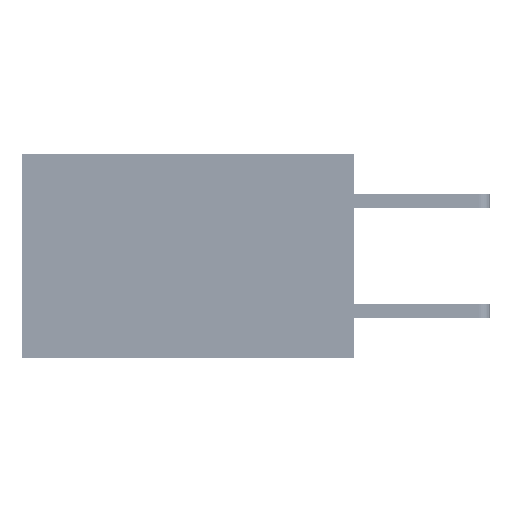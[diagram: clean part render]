
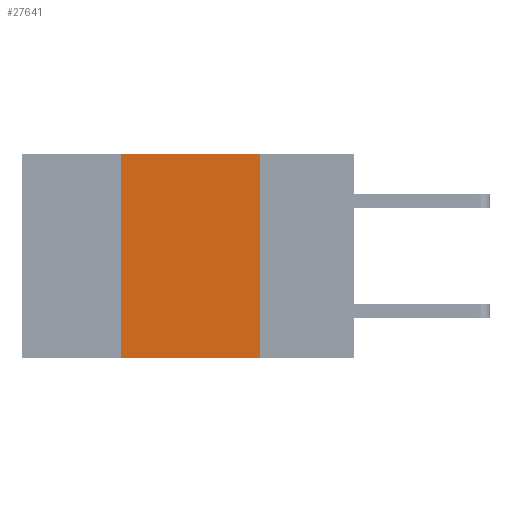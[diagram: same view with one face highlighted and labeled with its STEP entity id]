
A CAD part, left-side view. The second image highlights one B-rep face of the part: STEP entity #27641.
In plain terms, the highlighted planar face has unit normal (-1, 0, 0).
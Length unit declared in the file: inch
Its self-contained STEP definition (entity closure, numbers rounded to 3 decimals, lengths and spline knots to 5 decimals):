
#3107 = PLANE ( 'NONE',  #33369 ) ;
#4229 = ORIENTED_EDGE ( 'NONE', *, *, #21498, .F. ) ;
#5807 = EDGE_LOOP ( 'NONE', ( #47322, #31505, #4229, #15281 ) ) ;
#6145 = DIRECTION ( 'NONE',  ( 0., -1., 0. ) ) ;
#6495 = CARTESIAN_POINT ( 'NONE',  ( 0., 0.6, 0. ) ) ;
#8016 = VERTEX_POINT ( 'NONE', #31481 ) ;
#10145 = DIRECTION ( 'NONE',  ( 0., 0., -1. ) ) ;
#10960 = VERTEX_POINT ( 'NONE', #32849 ) ;
#13381 = DIRECTION ( 'NONE',  ( 0., -1., 0. ) ) ;
#15281 = ORIENTED_EDGE ( 'NONE', *, *, #38386, .T. ) ;
#15958 = DIRECTION ( 'NONE',  ( 0., 0., 1. ) ) ;
#18121 = CARTESIAN_POINT ( 'NONE',  ( 0., 0.17, -0.37 ) ) ;
#20200 = VECTOR ( 'NONE', #6145, 39.37008 ) ;
#21498 = EDGE_CURVE ( 'NONE', #10960, #31149, #31042, .T. ) ;
#22741 = VECTOR ( 'NONE', #13381, 39.37008 ) ;
#24629 = EDGE_CURVE ( 'NONE', #8016, #31662, #33028, .T. ) ;
#27272 = VECTOR ( 'NONE', #15958, 39.37008 ) ;
#27641 = ADVANCED_FACE ( 'NONE', ( #36888 ), #3107, .F. ) ;
#31042 = LINE ( 'NONE', #41758, #27272 ) ;
#31149 = VERTEX_POINT ( 'NONE', #43485 ) ;
#31481 = CARTESIAN_POINT ( 'NONE',  ( 0., 0.17, 0. ) ) ;
#31505 = ORIENTED_EDGE ( 'NONE', *, *, #43273, .F. ) ;
#31662 = VERTEX_POINT ( 'NONE', #18121 ) ;
#32849 = CARTESIAN_POINT ( 'NONE',  ( 0., 0.42, -0.37 ) ) ;
#33028 = LINE ( 'NONE', #43252, #37809 ) ;
#33369 = AXIS2_PLACEMENT_3D ( 'NONE', #6495, #44171, #10145 ) ;
#36546 = CARTESIAN_POINT ( 'NONE',  ( 0., 0.6, -0.37 ) ) ;
#36888 = FACE_OUTER_BOUND ( 'NONE', #5807, .T. ) ;
#37809 = VECTOR ( 'NONE', #47376, 39.37008 ) ;
#38386 = EDGE_CURVE ( 'NONE', #10960, #31662, #40200, .T. ) ;
#40200 = LINE ( 'NONE', #36546, #20200 ) ;
#41758 = CARTESIAN_POINT ( 'NONE',  ( 0., 0.42, 0. ) ) ;
#42575 = LINE ( 'NONE', #46453, #22741 ) ;
#43252 = CARTESIAN_POINT ( 'NONE',  ( 0., 0.17, 0. ) ) ;
#43273 = EDGE_CURVE ( 'NONE', #31149, #8016, #42575, .T. ) ;
#43485 = CARTESIAN_POINT ( 'NONE',  ( 0., 0.42, 0. ) ) ;
#44171 = DIRECTION ( 'NONE',  ( 1., 0., 0. ) ) ;
#46453 = CARTESIAN_POINT ( 'NONE',  ( 0., 0.6, 0. ) ) ;
#47322 = ORIENTED_EDGE ( 'NONE', *, *, #24629, .F. ) ;
#47376 = DIRECTION ( 'NONE',  ( 0., 0., -1. ) ) ;
